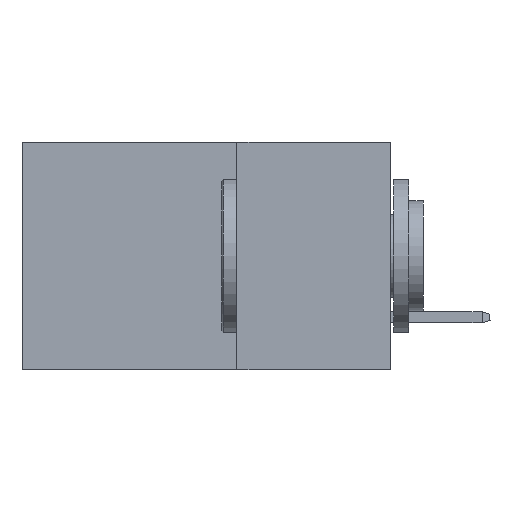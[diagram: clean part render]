
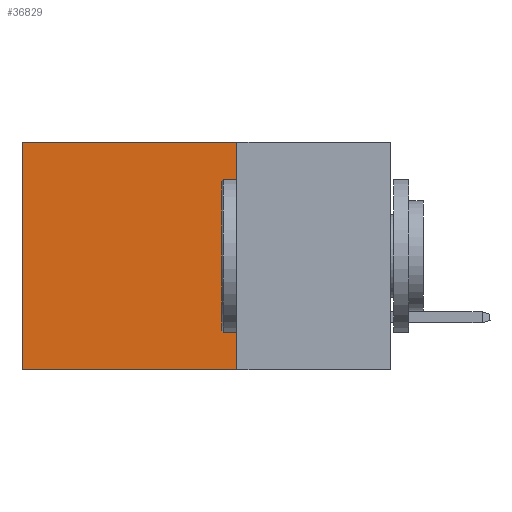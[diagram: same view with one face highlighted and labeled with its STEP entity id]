
A CAD part, left-side view. The second image highlights one B-rep face of the part: STEP entity #36829.
In plain terms, the highlighted planar face has unit normal (-1, 0, 0).
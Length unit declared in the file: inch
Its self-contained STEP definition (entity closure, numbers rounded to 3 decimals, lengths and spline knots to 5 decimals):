
#62 = AXIS2_PLACEMENT_3D ( 'NONE', #21940, #37922, #28818 ) ;
#802 = PLANE ( 'NONE',  #62 ) ;
#1856 = CARTESIAN_POINT ( 'NONE',  ( 0.2875, 0.25, 0. ) ) ;
#2748 = CARTESIAN_POINT ( 'NONE',  ( 0.2875, 0.25, 0. ) ) ;
#3414 = DIRECTION ( 'NONE',  ( 0., 0., -1. ) ) ;
#5599 = EDGE_LOOP ( 'NONE', ( #34073, #29995, #20923, #10504 ) ) ;
#5703 = CARTESIAN_POINT ( 'NONE',  ( 0.2875, 0.25, -0.37 ) ) ;
#8756 = EDGE_CURVE ( 'NONE', #14789, #35220, #35319, .T. ) ;
#8941 = CARTESIAN_POINT ( 'NONE',  ( 0.2875, 0.6, 0. ) ) ;
#9577 = VECTOR ( 'NONE', #23618, 39.37008 ) ;
#10504 = ORIENTED_EDGE ( 'NONE', *, *, #8756, .T. ) ;
#11496 = LINE ( 'NONE', #26384, #9577 ) ;
#11818 = DIRECTION ( 'NONE',  ( 0., 1., 0. ) ) ;
#14094 = VERTEX_POINT ( 'NONE', #5703 ) ;
#14101 = FACE_OUTER_BOUND ( 'NONE', #5599, .T. ) ;
#14789 = VERTEX_POINT ( 'NONE', #1856 ) ;
#15133 = CARTESIAN_POINT ( 'NONE',  ( 0.2875, 0.6, -0.37 ) ) ;
#16307 = EDGE_CURVE ( 'NONE', #14789, #14094, #11496, .T. ) ;
#16408 = VECTOR ( 'NONE', #26457, 39.37008 ) ;
#17148 = VERTEX_POINT ( 'NONE', #15133 ) ;
#17521 = LINE ( 'NONE', #30828, #29360 ) ;
#20923 = ORIENTED_EDGE ( 'NONE', *, *, #16307, .F. ) ;
#21940 = CARTESIAN_POINT ( 'NONE',  ( 0.2875, 0.25, 0. ) ) ;
#23618 = DIRECTION ( 'NONE',  ( 0., 0., -1. ) ) ;
#23902 = EDGE_CURVE ( 'NONE', #35220, #17148, #17521, .T. ) ;
#24470 = LINE ( 'NONE', #32403, #16408 ) ;
#25523 = EDGE_CURVE ( 'NONE', #14094, #17148, #24470, .T. ) ;
#26384 = CARTESIAN_POINT ( 'NONE',  ( 0.2875, 0.25, 0. ) ) ;
#26457 = DIRECTION ( 'NONE',  ( 0., 1., 0. ) ) ;
#28818 = DIRECTION ( 'NONE',  ( 0., 0., -1. ) ) ;
#29360 = VECTOR ( 'NONE', #3414, 39.37008 ) ;
#29995 = ORIENTED_EDGE ( 'NONE', *, *, #25523, .F. ) ;
#30545 = VECTOR ( 'NONE', #11818, 39.37008 ) ;
#30828 = CARTESIAN_POINT ( 'NONE',  ( 0.2875, 0.6, 0. ) ) ;
#32403 = CARTESIAN_POINT ( 'NONE',  ( 0.2875, 0.25, -0.37 ) ) ;
#34073 = ORIENTED_EDGE ( 'NONE', *, *, #23902, .T. ) ;
#35220 = VERTEX_POINT ( 'NONE', #8941 ) ;
#35319 = LINE ( 'NONE', #2748, #30545 ) ;
#36829 = ADVANCED_FACE ( 'NONE', ( #14101 ), #802, .F. ) ;
#37922 = DIRECTION ( 'NONE',  ( 1., 0., 0. ) ) ;
